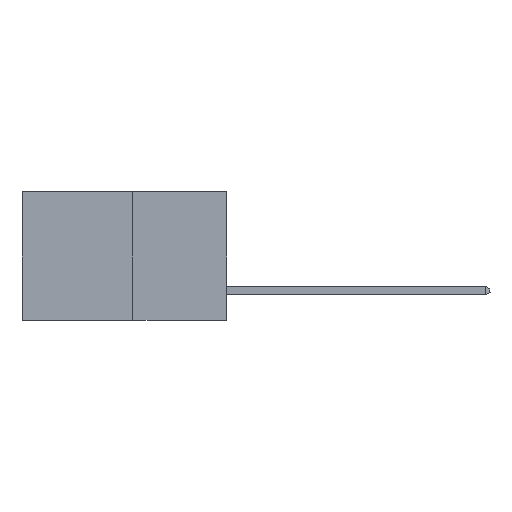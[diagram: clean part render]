
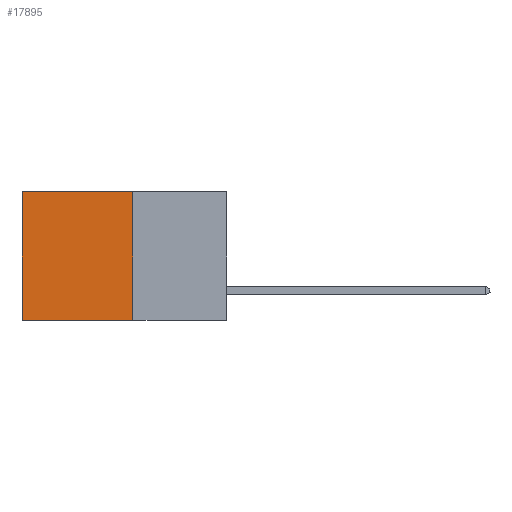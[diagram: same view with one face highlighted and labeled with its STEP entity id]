
A CAD part, left-side view. The second image highlights one B-rep face of the part: STEP entity #17895.
In plain terms, the highlighted planar face has unit normal (-1, 0, 0).
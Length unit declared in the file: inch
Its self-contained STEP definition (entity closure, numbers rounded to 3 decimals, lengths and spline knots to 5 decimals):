
#822 = CARTESIAN_POINT ( 'NONE',  ( 0.277, 0.27, 0. ) ) ;
#1516 = PLANE ( 'NONE',  #9113 ) ;
#1733 = VECTOR ( 'NONE', #20444, 39.37008 ) ;
#2662 = EDGE_LOOP ( 'NONE', ( #3673, #16035, #16648, #21929 ) ) ;
#3445 = VERTEX_POINT ( 'NONE', #19848 ) ;
#3673 = ORIENTED_EDGE ( 'NONE', *, *, #4800, .T. ) ;
#4376 = EDGE_CURVE ( 'NONE', #20087, #3445, #10501, .T. ) ;
#4780 = CARTESIAN_POINT ( 'NONE',  ( 0.277, 0.59, -0.37 ) ) ;
#4800 = EDGE_CURVE ( 'NONE', #7632, #3445, #20119, .T. ) ;
#5366 = DIRECTION ( 'NONE',  ( 1., 0., 0. ) ) ;
#6984 = VERTEX_POINT ( 'NONE', #822 ) ;
#7632 = VERTEX_POINT ( 'NONE', #13101 ) ;
#7759 = DIRECTION ( 'NONE',  ( 0., 0., -1. ) ) ;
#7991 = DIRECTION ( 'NONE',  ( 0., 1., 0. ) ) ;
#9113 = AXIS2_PLACEMENT_3D ( 'NONE', #16339, #5366, #18146 ) ;
#10501 = LINE ( 'NONE', #12141, #15942 ) ;
#12141 = CARTESIAN_POINT ( 'NONE',  ( 0.277, 0.27, -0.37 ) ) ;
#12365 = VECTOR ( 'NONE', #7759, 39.37008 ) ;
#12643 = LINE ( 'NONE', #17425, #18044 ) ;
#13101 = CARTESIAN_POINT ( 'NONE',  ( 0.277, 0.59, 0. ) ) ;
#15063 = CARTESIAN_POINT ( 'NONE',  ( 0.277, 0.27, -0.37 ) ) ;
#15942 = VECTOR ( 'NONE', #7991, 39.37008 ) ;
#16035 = ORIENTED_EDGE ( 'NONE', *, *, #4376, .F. ) ;
#16339 = CARTESIAN_POINT ( 'NONE',  ( 0.277, 0.27, -0.37 ) ) ;
#16648 = ORIENTED_EDGE ( 'NONE', *, *, #18083, .F. ) ;
#17225 = LINE ( 'NONE', #15063, #12365 ) ;
#17425 = CARTESIAN_POINT ( 'NONE',  ( 0.277, 0.27, 0. ) ) ;
#17895 = ADVANCED_FACE ( 'NONE', ( #21675 ), #1516, .F. ) ;
#18044 = VECTOR ( 'NONE', #19215, 39.37008 ) ;
#18083 = EDGE_CURVE ( 'NONE', #6984, #20087, #17225, .T. ) ;
#18146 = DIRECTION ( 'NONE',  ( 0., 0., -1. ) ) ;
#18285 = EDGE_CURVE ( 'NONE', #6984, #7632, #12643, .T. ) ;
#19215 = DIRECTION ( 'NONE',  ( 0., 1., 0. ) ) ;
#19848 = CARTESIAN_POINT ( 'NONE',  ( 0.277, 0.59, -0.37 ) ) ;
#20087 = VERTEX_POINT ( 'NONE', #22459 ) ;
#20119 = LINE ( 'NONE', #4780, #1733 ) ;
#20444 = DIRECTION ( 'NONE',  ( 0., 0., -1. ) ) ;
#21675 = FACE_OUTER_BOUND ( 'NONE', #2662, .T. ) ;
#21929 = ORIENTED_EDGE ( 'NONE', *, *, #18285, .T. ) ;
#22459 = CARTESIAN_POINT ( 'NONE',  ( 0.277, 0.27, -0.37 ) ) ;
